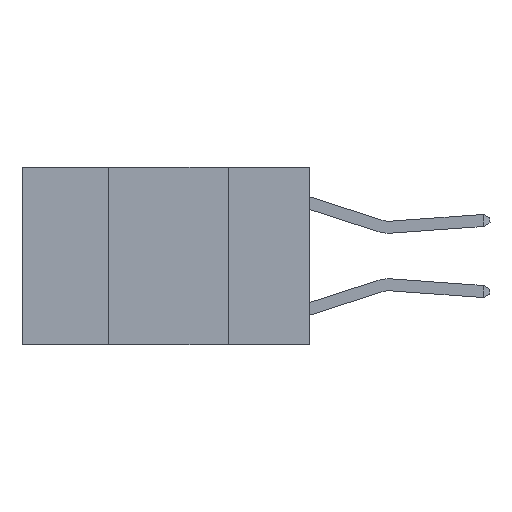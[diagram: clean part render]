
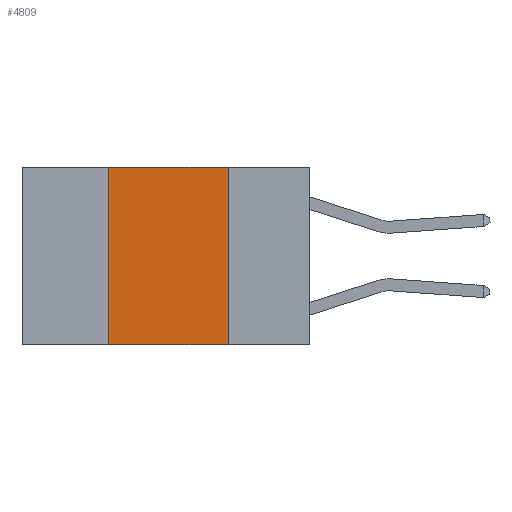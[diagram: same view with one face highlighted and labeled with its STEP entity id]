
A CAD part, left-side view. The second image highlights one B-rep face of the part: STEP entity #4809.
In plain terms, the highlighted planar face has unit normal (-1, 0, 0).
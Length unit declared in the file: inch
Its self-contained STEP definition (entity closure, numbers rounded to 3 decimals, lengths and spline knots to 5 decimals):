
#223 = LINE ( 'NONE', #21003, #23228 ) ;
#404 = CARTESIAN_POINT ( 'NONE',  ( 0., 0.6, 0. ) ) ;
#712 = ORIENTED_EDGE ( 'NONE', *, *, #3873, .F. ) ;
#922 = ORIENTED_EDGE ( 'NONE', *, *, #3414, .F. ) ;
#1017 = VERTEX_POINT ( 'NONE', #13995 ) ;
#1176 = ORIENTED_EDGE ( 'NONE', *, *, #7400, .T. ) ;
#1244 = DIRECTION ( 'NONE',  ( 1., 0., 0. ) ) ;
#1564 = CARTESIAN_POINT ( 'NONE',  ( 0., 0.42, 0. ) ) ;
#1648 = FACE_OUTER_BOUND ( 'NONE', #16043, .T. ) ;
#1985 = AXIS2_PLACEMENT_3D ( 'NONE', #12256, #1244, #14097 ) ;
#2253 = DIRECTION ( 'NONE',  ( 0., -1., 0. ) ) ;
#2837 = DIRECTION ( 'NONE',  ( 0., 0., 1. ) ) ;
#3414 = EDGE_CURVE ( 'NONE', #1017, #16174, #223, .T. ) ;
#3873 = EDGE_CURVE ( 'NONE', #16174, #20400, #5423, .T. ) ;
#4013 = CARTESIAN_POINT ( 'NONE',  ( 0., 0.6, -0.37 ) ) ;
#4587 = VECTOR ( 'NONE', #12450, 39.37008 ) ;
#4809 = ADVANCED_FACE ( 'NONE', ( #1648 ), #23005, .F. ) ;
#5423 = LINE ( 'NONE', #404, #14603 ) ;
#7400 = EDGE_CURVE ( 'NONE', #1017, #12390, #18409, .T. ) ;
#8890 = CARTESIAN_POINT ( 'NONE',  ( 0., 0.17, 0. ) ) ;
#9275 = VECTOR ( 'NONE', #16817, 39.37008 ) ;
#9860 = ORIENTED_EDGE ( 'NONE', *, *, #11275, .F. ) ;
#10603 = CARTESIAN_POINT ( 'NONE',  ( 0., 0.17, 0. ) ) ;
#11275 = EDGE_CURVE ( 'NONE', #20400, #12390, #19154, .T. ) ;
#12256 = CARTESIAN_POINT ( 'NONE',  ( 0., 0.6, 0. ) ) ;
#12390 = VERTEX_POINT ( 'NONE', #18891 ) ;
#12450 = DIRECTION ( 'NONE',  ( 0., 0., -1. ) ) ;
#13995 = CARTESIAN_POINT ( 'NONE',  ( 0., 0.42, -0.37 ) ) ;
#14097 = DIRECTION ( 'NONE',  ( 0., 0., -1. ) ) ;
#14603 = VECTOR ( 'NONE', #2253, 39.37008 ) ;
#16043 = EDGE_LOOP ( 'NONE', ( #9860, #712, #922, #1176 ) ) ;
#16174 = VERTEX_POINT ( 'NONE', #1564 ) ;
#16817 = DIRECTION ( 'NONE',  ( 0., -1., 0. ) ) ;
#18409 = LINE ( 'NONE', #4013, #9275 ) ;
#18891 = CARTESIAN_POINT ( 'NONE',  ( 0., 0.17, -0.37 ) ) ;
#19154 = LINE ( 'NONE', #10603, #4587 ) ;
#20400 = VERTEX_POINT ( 'NONE', #8890 ) ;
#21003 = CARTESIAN_POINT ( 'NONE',  ( 0., 0.42, 0. ) ) ;
#23005 = PLANE ( 'NONE',  #1985 ) ;
#23228 = VECTOR ( 'NONE', #2837, 39.37008 ) ;
